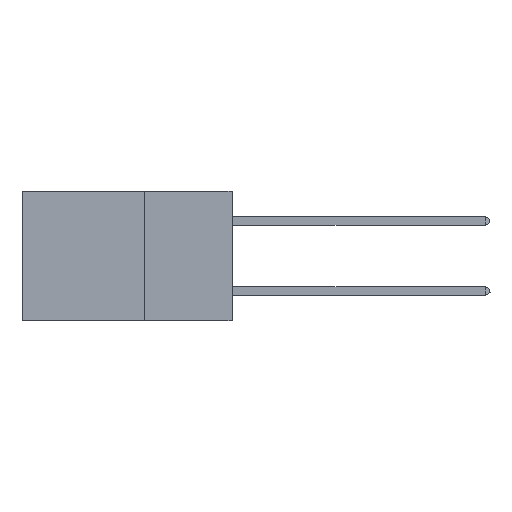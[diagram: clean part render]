
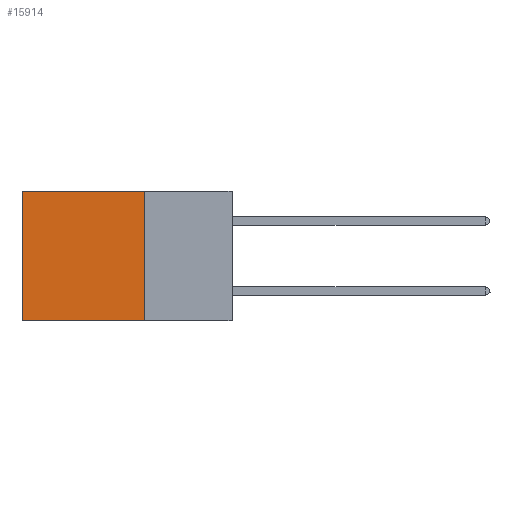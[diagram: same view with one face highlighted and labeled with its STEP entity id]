
A CAD part, left-side view. The second image highlights one B-rep face of the part: STEP entity #15914.
In plain terms, the highlighted planar face has unit normal (-1, 0, 0).
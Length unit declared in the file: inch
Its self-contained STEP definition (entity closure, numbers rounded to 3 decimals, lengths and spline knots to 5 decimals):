
#151 = DIRECTION ( 'NONE',  ( 0., 0., -1. ) ) ;
#2315 = LINE ( 'NONE', #4987, #18288 ) ;
#2983 = VERTEX_POINT ( 'NONE', #6001 ) ;
#3297 = DIRECTION ( 'NONE',  ( 0., 1., 0. ) ) ;
#3399 = ORIENTED_EDGE ( 'NONE', *, *, #6410, .F. ) ;
#4987 = CARTESIAN_POINT ( 'NONE',  ( 0.2875, 0.25, 0. ) ) ;
#5824 = FACE_OUTER_BOUND ( 'NONE', #21389, .T. ) ;
#5963 = DIRECTION ( 'NONE',  ( 0., 0., -1. ) ) ;
#6001 = CARTESIAN_POINT ( 'NONE',  ( 0.2875, 0.25, -0.37 ) ) ;
#6159 = ORIENTED_EDGE ( 'NONE', *, *, #12268, .T. ) ;
#6368 = VECTOR ( 'NONE', #10257, 39.37008 ) ;
#6410 = EDGE_CURVE ( 'NONE', #2983, #9412, #17669, .T. ) ;
#6441 = LINE ( 'NONE', #16255, #13443 ) ;
#7685 = CARTESIAN_POINT ( 'NONE',  ( 0.2875, 0.25, 0. ) ) ;
#8513 = VERTEX_POINT ( 'NONE', #12030 ) ;
#9412 = VERTEX_POINT ( 'NONE', #12808 ) ;
#10257 = DIRECTION ( 'NONE',  ( 0., 1., 0. ) ) ;
#10708 = DIRECTION ( 'NONE',  ( 1., 0., 0. ) ) ;
#11417 = DIRECTION ( 'NONE',  ( 0., 0., -1. ) ) ;
#12010 = EDGE_CURVE ( 'NONE', #8513, #9412, #6441, .T. ) ;
#12030 = CARTESIAN_POINT ( 'NONE',  ( 0.2875, 0.6, 0. ) ) ;
#12268 = EDGE_CURVE ( 'NONE', #17648, #8513, #2315, .T. ) ;
#12551 = ORIENTED_EDGE ( 'NONE', *, *, #17406, .F. ) ;
#12808 = CARTESIAN_POINT ( 'NONE',  ( 0.2875, 0.6, -0.37 ) ) ;
#13443 = VECTOR ( 'NONE', #5963, 39.37008 ) ;
#14058 = PLANE ( 'NONE',  #19056 ) ;
#15914 = ADVANCED_FACE ( 'NONE', ( #5824 ), #14058, .F. ) ;
#16017 = ORIENTED_EDGE ( 'NONE', *, *, #12010, .T. ) ;
#16036 = LINE ( 'NONE', #7685, #16314 ) ;
#16255 = CARTESIAN_POINT ( 'NONE',  ( 0.2875, 0.6, 0. ) ) ;
#16314 = VECTOR ( 'NONE', #11417, 39.37008 ) ;
#17406 = EDGE_CURVE ( 'NONE', #17648, #2983, #16036, .T. ) ;
#17648 = VERTEX_POINT ( 'NONE', #18706 ) ;
#17669 = LINE ( 'NONE', #19035, #6368 ) ;
#18288 = VECTOR ( 'NONE', #3297, 39.37008 ) ;
#18706 = CARTESIAN_POINT ( 'NONE',  ( 0.2875, 0.25, 0. ) ) ;
#19035 = CARTESIAN_POINT ( 'NONE',  ( 0.2875, 0.25, -0.37 ) ) ;
#19056 = AXIS2_PLACEMENT_3D ( 'NONE', #19076, #10708, #151 ) ;
#19076 = CARTESIAN_POINT ( 'NONE',  ( 0.2875, 0.25, 0. ) ) ;
#21389 = EDGE_LOOP ( 'NONE', ( #16017, #3399, #12551, #6159 ) ) ;
